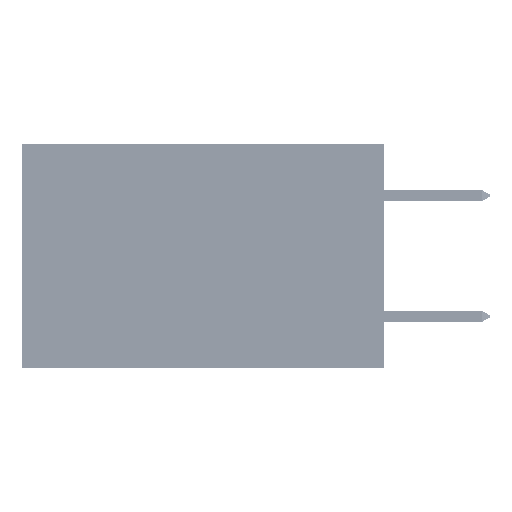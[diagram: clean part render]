
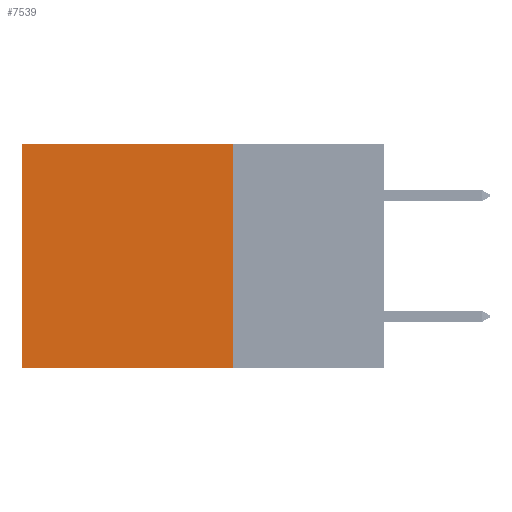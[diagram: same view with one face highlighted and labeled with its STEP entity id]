
A CAD part, left-side view. The second image highlights one B-rep face of the part: STEP entity #7539.
In plain terms, the highlighted planar face has unit normal (-1, 0, 0).
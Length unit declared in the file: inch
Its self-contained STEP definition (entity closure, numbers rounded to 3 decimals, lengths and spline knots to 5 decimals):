
#4989 = PLANE ( 'NONE',  #37914 ) ;
#5797 = CARTESIAN_POINT ( 'NONE',  ( 0.2875, 0.6, -0.37 ) ) ;
#6802 = ORIENTED_EDGE ( 'NONE', *, *, #17838, .T. ) ;
#7442 = CARTESIAN_POINT ( 'NONE',  ( 0.2875, 0.25, 0. ) ) ;
#7479 = EDGE_LOOP ( 'NONE', ( #19271, #40049, #24959, #6802 ) ) ;
#7539 = ADVANCED_FACE ( 'NONE', ( #11395 ), #4989, .F. ) ;
#7616 = LINE ( 'NONE', #22642, #33607 ) ;
#8007 = VECTOR ( 'NONE', #48162, 39.37008 ) ;
#9140 = DIRECTION ( 'NONE',  ( 1., 0., 0. ) ) ;
#11262 = VECTOR ( 'NONE', #31787, 39.37008 ) ;
#11395 = FACE_OUTER_BOUND ( 'NONE', #7479, .T. ) ;
#11844 = EDGE_CURVE ( 'NONE', #31040, #25527, #31640, .T. ) ;
#13520 = EDGE_CURVE ( 'NONE', #28523, #31040, #36524, .T. ) ;
#14584 = DIRECTION ( 'NONE',  ( 0., 1., 0. ) ) ;
#17634 = VERTEX_POINT ( 'NONE', #36883 ) ;
#17838 = EDGE_CURVE ( 'NONE', #28523, #17634, #7616, .T. ) ;
#19271 = ORIENTED_EDGE ( 'NONE', *, *, #39034, .T. ) ;
#22642 = CARTESIAN_POINT ( 'NONE',  ( 0.2875, 0.25, 0. ) ) ;
#24959 = ORIENTED_EDGE ( 'NONE', *, *, #13520, .F. ) ;
#25527 = VERTEX_POINT ( 'NONE', #5797 ) ;
#28523 = VERTEX_POINT ( 'NONE', #31079 ) ;
#29166 = VECTOR ( 'NONE', #14584, 39.37008 ) ;
#31040 = VERTEX_POINT ( 'NONE', #50767 ) ;
#31079 = CARTESIAN_POINT ( 'NONE',  ( 0.2875, 0.25, 0. ) ) ;
#31450 = CARTESIAN_POINT ( 'NONE',  ( 0.2875, 0.6, 0. ) ) ;
#31640 = LINE ( 'NONE', #46479, #29166 ) ;
#31787 = DIRECTION ( 'NONE',  ( 0., 0., -1. ) ) ;
#32830 = CARTESIAN_POINT ( 'NONE',  ( 0.2875, 0.25, 0. ) ) ;
#33338 = DIRECTION ( 'NONE',  ( 0., 0., -1. ) ) ;
#33607 = VECTOR ( 'NONE', #50399, 39.37008 ) ;
#36524 = LINE ( 'NONE', #7442, #8007 ) ;
#36883 = CARTESIAN_POINT ( 'NONE',  ( 0.2875, 0.6, 0. ) ) ;
#37914 = AXIS2_PLACEMENT_3D ( 'NONE', #32830, #9140, #33338 ) ;
#39034 = EDGE_CURVE ( 'NONE', #17634, #25527, #46644, .T. ) ;
#40049 = ORIENTED_EDGE ( 'NONE', *, *, #11844, .F. ) ;
#46479 = CARTESIAN_POINT ( 'NONE',  ( 0.2875, 0.25, -0.37 ) ) ;
#46644 = LINE ( 'NONE', #31450, #11262 ) ;
#48162 = DIRECTION ( 'NONE',  ( 0., 0., -1. ) ) ;
#50399 = DIRECTION ( 'NONE',  ( 0., 1., 0. ) ) ;
#50767 = CARTESIAN_POINT ( 'NONE',  ( 0.2875, 0.25, -0.37 ) ) ;
